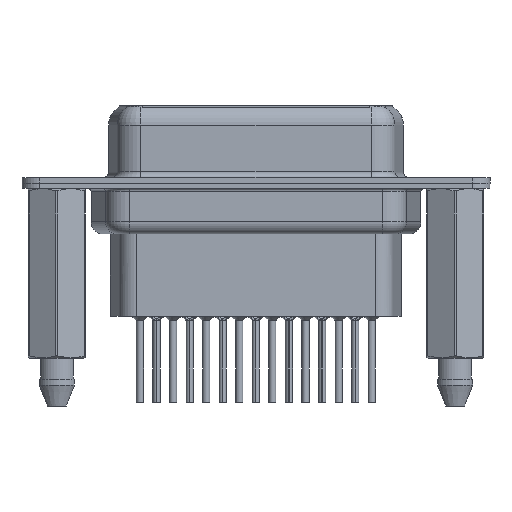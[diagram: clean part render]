
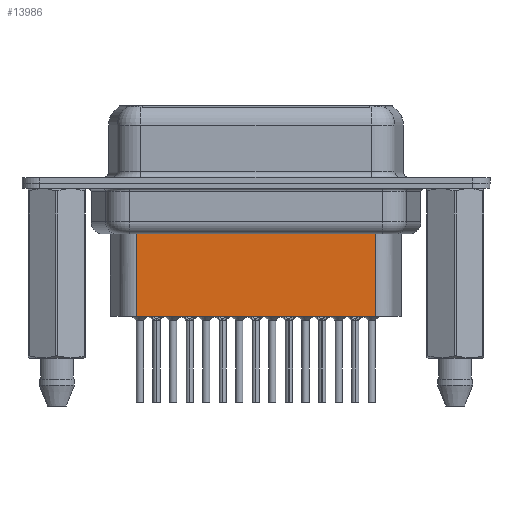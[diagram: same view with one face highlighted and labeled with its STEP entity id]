
A CAD part, front view. The second image highlights one B-rep face of the part: STEP entity #13986.
In plain terms, the highlighted planar face has unit normal (0, -1, 0).
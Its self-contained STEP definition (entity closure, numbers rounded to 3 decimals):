
#339 = ORIENTED_EDGE ( 'NONE', *, *, #15671, .F. ) ;
#941 = VECTOR ( 'NONE', #22973, 1000. ) ;
#968 = VERTEX_POINT ( 'NONE', #17149 ) ;
#1229 = PLANE ( 'NONE',  #13441 ) ;
#4237 = EDGE_CURVE ( 'NONE', #22286, #5791, #17626, .T. ) ;
#5097 = DIRECTION ( 'NONE',  ( 0., 0., -1. ) ) ;
#5791 = VERTEX_POINT ( 'NONE', #20282 ) ;
#5934 = ORIENTED_EDGE ( 'NONE', *, *, #16729, .T. ) ;
#6973 = ORIENTED_EDGE ( 'NONE', *, *, #4237, .T. ) ;
#7892 = DIRECTION ( 'NONE',  ( -1., 0., 0. ) ) ;
#10497 = CARTESIAN_POINT ( 'NONE',  ( 26.619, -3.5, -4.097 ) ) ;
#12067 = DIRECTION ( 'NONE',  ( 0., 0., -1. ) ) ;
#12223 = VERTEX_POINT ( 'NONE', #20630 ) ;
#12586 = ORIENTED_EDGE ( 'NONE', *, *, #24556, .F. ) ;
#13441 = AXIS2_PLACEMENT_3D ( 'NONE', #24747, #15087, #22966 ) ;
#13623 = LINE ( 'NONE', #21625, #22087 ) ;
#13986 = ADVANCED_FACE ( 'NONE', ( #18794 ), #1229, .T. ) ;
#14148 = CARTESIAN_POINT ( 'NONE',  ( 6.434, -3.5, -4.097 ) ) ;
#14784 = VECTOR ( 'NONE', #7892, 1000. ) ;
#15087 = DIRECTION ( 'NONE',  ( 0., -1., 0. ) ) ;
#15152 = LINE ( 'NONE', #20761, #20650 ) ;
#15217 = CARTESIAN_POINT ( 'NONE',  ( 6.681, -3.5, -11.15 ) ) ;
#15671 = EDGE_CURVE ( 'NONE', #12223, #968, #17169, .T. ) ;
#16729 = EDGE_CURVE ( 'NONE', #5791, #968, #13623, .T. ) ;
#17149 = CARTESIAN_POINT ( 'NONE',  ( 6.681, -3.5, -11.15 ) ) ;
#17169 = LINE ( 'NONE', #15217, #941 ) ;
#17626 = LINE ( 'NONE', #14148, #14784 ) ;
#18794 = FACE_OUTER_BOUND ( 'NONE', #20651, .T. ) ;
#20282 = CARTESIAN_POINT ( 'NONE',  ( 6.681, -3.5, -4.097 ) ) ;
#20630 = CARTESIAN_POINT ( 'NONE',  ( 26.619, -3.5, -11.15 ) ) ;
#20650 = VECTOR ( 'NONE', #5097, 1000. ) ;
#20651 = EDGE_LOOP ( 'NONE', ( #12586, #6973, #5934, #339 ) ) ;
#20761 = CARTESIAN_POINT ( 'NONE',  ( 26.619, -3.5, -3.1 ) ) ;
#21625 = CARTESIAN_POINT ( 'NONE',  ( 6.681, -3.5, -3.1 ) ) ;
#22087 = VECTOR ( 'NONE', #12067, 1000. ) ;
#22286 = VERTEX_POINT ( 'NONE', #10497 ) ;
#22966 = DIRECTION ( 'NONE',  ( 1., 0., 0. ) ) ;
#22973 = DIRECTION ( 'NONE',  ( -1., 0., 0. ) ) ;
#24556 = EDGE_CURVE ( 'NONE', #22286, #12223, #15152, .T. ) ;
#24747 = CARTESIAN_POINT ( 'NONE',  ( 6.681, -3.5, -3.1 ) ) ;
